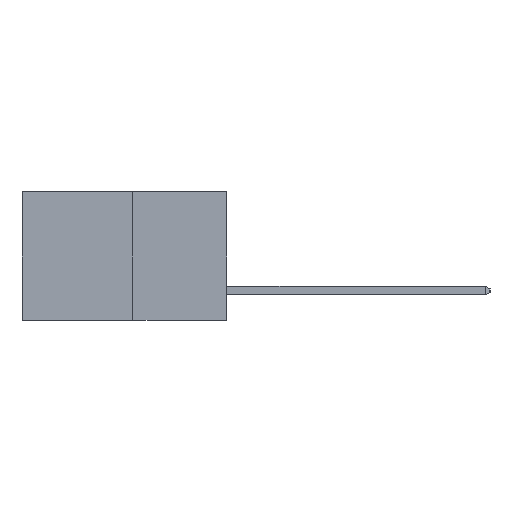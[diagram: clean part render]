
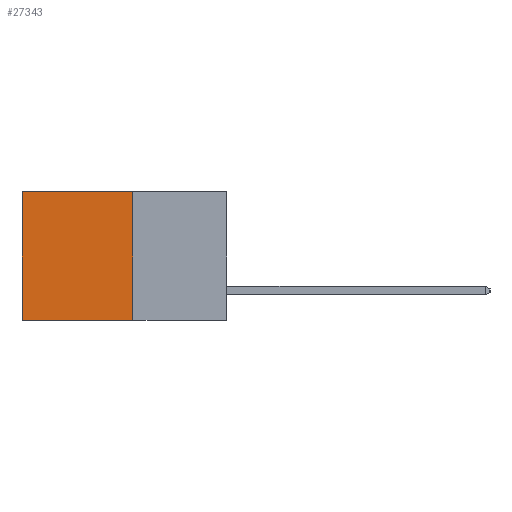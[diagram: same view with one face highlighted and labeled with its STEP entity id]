
A CAD part, left-side view. The second image highlights one B-rep face of the part: STEP entity #27343.
In plain terms, the highlighted planar face has unit normal (-1, 0, 0).
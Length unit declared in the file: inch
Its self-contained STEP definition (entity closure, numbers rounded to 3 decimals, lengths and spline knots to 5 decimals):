
#462 = EDGE_LOOP ( 'NONE', ( #19318, #20330, #13415, #3389 ) ) ;
#1968 = DIRECTION ( 'NONE',  ( 0., 0., -1. ) ) ;
#3389 = ORIENTED_EDGE ( 'NONE', *, *, #18276, .T. ) ;
#4497 = LINE ( 'NONE', #12331, #22550 ) ;
#6843 = EDGE_CURVE ( 'NONE', #21933, #24439, #26722, .T. ) ;
#6886 = DIRECTION ( 'NONE',  ( 0., 1., 0. ) ) ;
#6992 = VERTEX_POINT ( 'NONE', #19881 ) ;
#10734 = CARTESIAN_POINT ( 'NONE',  ( 0.277, 0.27, -0.37 ) ) ;
#10748 = DIRECTION ( 'NONE',  ( 0., 0., -1. ) ) ;
#12331 = CARTESIAN_POINT ( 'NONE',  ( 0.277, 0.27, 0. ) ) ;
#12919 = DIRECTION ( 'NONE',  ( 0., 0., -1. ) ) ;
#13380 = EDGE_CURVE ( 'NONE', #24088, #6992, #24449, .T. ) ;
#13415 = ORIENTED_EDGE ( 'NONE', *, *, #6843, .F. ) ;
#14497 = DIRECTION ( 'NONE',  ( 0., 1., 0. ) ) ;
#14521 = VECTOR ( 'NONE', #6886, 39.37008 ) ;
#17736 = CARTESIAN_POINT ( 'NONE',  ( 0.277, 0.27, -0.37 ) ) ;
#18276 = EDGE_CURVE ( 'NONE', #21933, #24088, #4497, .T. ) ;
#18686 = VECTOR ( 'NONE', #10748, 39.37008 ) ;
#19318 = ORIENTED_EDGE ( 'NONE', *, *, #13380, .T. ) ;
#19881 = CARTESIAN_POINT ( 'NONE',  ( 0.277, 0.59, -0.37 ) ) ;
#19893 = AXIS2_PLACEMENT_3D ( 'NONE', #10734, #25921, #12919 ) ;
#20330 = ORIENTED_EDGE ( 'NONE', *, *, #23768, .F. ) ;
#20384 = CARTESIAN_POINT ( 'NONE',  ( 0.277, 0.27, -0.37 ) ) ;
#20964 = CARTESIAN_POINT ( 'NONE',  ( 0.277, 0.59, 0. ) ) ;
#20983 = VECTOR ( 'NONE', #1968, 39.37008 ) ;
#21572 = PLANE ( 'NONE',  #19893 ) ;
#21586 = CARTESIAN_POINT ( 'NONE',  ( 0.277, 0.59, -0.37 ) ) ;
#21933 = VERTEX_POINT ( 'NONE', #22017 ) ;
#22017 = CARTESIAN_POINT ( 'NONE',  ( 0.277, 0.27, 0. ) ) ;
#22550 = VECTOR ( 'NONE', #14497, 39.37008 ) ;
#23768 = EDGE_CURVE ( 'NONE', #24439, #6992, #26741, .T. ) ;
#24088 = VERTEX_POINT ( 'NONE', #20964 ) ;
#24439 = VERTEX_POINT ( 'NONE', #20384 ) ;
#24449 = LINE ( 'NONE', #21586, #18686 ) ;
#24544 = FACE_OUTER_BOUND ( 'NONE', #462, .T. ) ;
#25921 = DIRECTION ( 'NONE',  ( 1., 0., 0. ) ) ;
#26722 = LINE ( 'NONE', #28244, #20983 ) ;
#26741 = LINE ( 'NONE', #17736, #14521 ) ;
#27343 = ADVANCED_FACE ( 'NONE', ( #24544 ), #21572, .F. ) ;
#28244 = CARTESIAN_POINT ( 'NONE',  ( 0.277, 0.27, -0.37 ) ) ;
